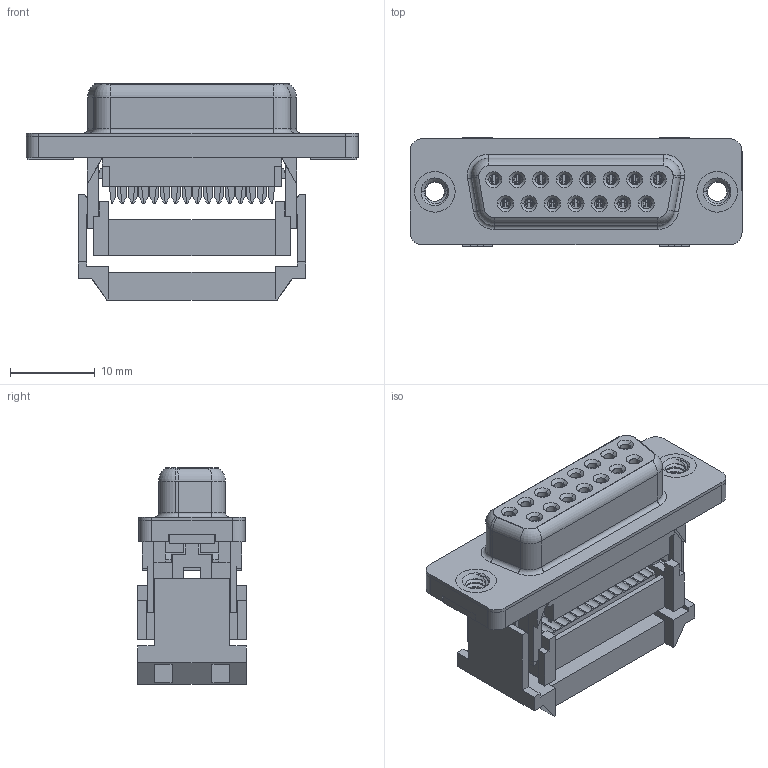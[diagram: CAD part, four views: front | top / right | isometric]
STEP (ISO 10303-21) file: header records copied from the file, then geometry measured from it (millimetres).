
FILE_DESCRIPTION (( 'STEP AP203' ), '1' );
FILE_NAME ('628-015-327-012.STEP', '2020-07-16T13:45:43', ( '' ), ( '' ), 'SwSTEP 2.0', 'SolidWorks 2020', '' );
FILE_SCHEMA (( 'CONFIG_CONTROL_DESIGN' ));
Length unit declared in the file: millimetre
Products named in the file (8): 628 IDC Contacts_15 Contacts; 628 IDC 4-40 Threaded Rivet; 628 IDC Cable Cover_15 Contacts; 628 PB Shell_15 Contacts; 628-015-327-012; 628 IDC Housing_15 Contacts; 628 IDC Guide Front_15 Contacts; 628 IDC Guide Rear_15 Contacts
Assembly tree (8 placements, depth 2):
  628-015-327-012
    628 IDC Housing_15 Contacts
    628 IDC Guide Front_15 Contacts
    628 IDC Guide Rear_15 Contacts
    628 IDC Cable Cover_15 Contacts
    628 PB Shell_15 Contacts
    628 IDC Contacts_15 Contacts
    628 IDC 4-40 Threaded Rivet  x2
Bounding box: 39.19 x 12.85 x 25.5 mm (x, y, z)
Volume: 4329.5 mm3; surface area: 8969.5 mm2
Topology: 24 solids, 24 shells, 2629 faces, 6695 edges, 4142 vertices
Faces by surface type: plane 1588, cylinder 557, torus 273, cone 190, bspline 21
Entity records: 80062 total; most frequent: CARTESIAN_POINT 15546, DIRECTION 13451, ORIENTED_EDGE 13240, EDGE_CURVE 6620, VECTOR 4707, LINE 4707, AXIS2_PLACEMENT_3D 4372, VERTEX_POINT 4093
